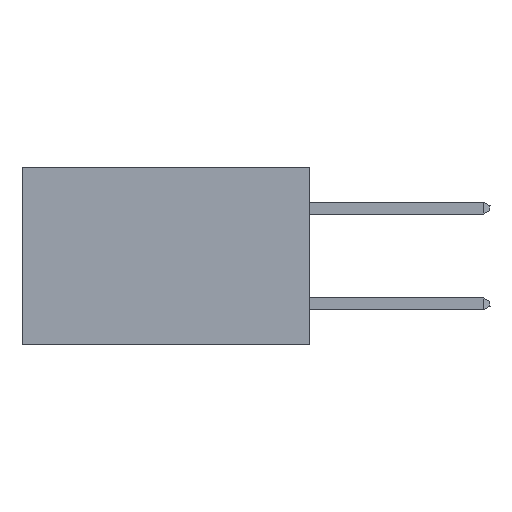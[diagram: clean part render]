
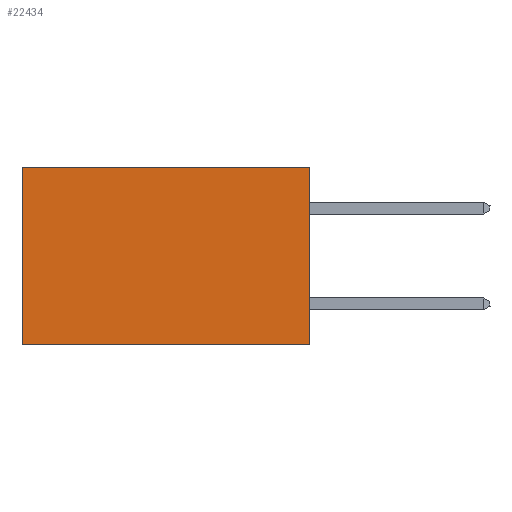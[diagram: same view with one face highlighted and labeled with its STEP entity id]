
A CAD part, left-side view. The second image highlights one B-rep face of the part: STEP entity #22434.
In plain terms, the highlighted planar face has unit normal (-1, 0, 0).
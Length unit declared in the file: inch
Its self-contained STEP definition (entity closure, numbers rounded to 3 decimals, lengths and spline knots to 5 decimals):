
#563 = AXIS2_PLACEMENT_3D ( 'NONE', #19935, #7311, #22118 ) ;
#1279 = CARTESIAN_POINT ( 'NONE',  ( 0.2875, 0.6, 0. ) ) ;
#1547 = DIRECTION ( 'NONE',  ( 0., 0., -1. ) ) ;
#2875 = DIRECTION ( 'NONE',  ( 0., 1., 0. ) ) ;
#2986 = FACE_OUTER_BOUND ( 'NONE', #8673, .T. ) ;
#3261 = LINE ( 'NONE', #4992, #24532 ) ;
#4283 = ORIENTED_EDGE ( 'NONE', *, *, #12725, .F. ) ;
#4875 = CARTESIAN_POINT ( 'NONE',  ( 0.2875, 0., -0.37 ) ) ;
#4992 = CARTESIAN_POINT ( 'NONE',  ( 0.2875, 0., 0. ) ) ;
#5690 = DIRECTION ( 'NONE',  ( 0., 0., -1. ) ) ;
#6287 = CARTESIAN_POINT ( 'NONE',  ( 0.2875, 0., 0. ) ) ;
#6852 = VERTEX_POINT ( 'NONE', #23086 ) ;
#7311 = DIRECTION ( 'NONE',  ( 1., 0., 0. ) ) ;
#7563 = VECTOR ( 'NONE', #5690, 39.37008 ) ;
#8171 = ORIENTED_EDGE ( 'NONE', *, *, #17088, .F. ) ;
#8196 = CARTESIAN_POINT ( 'NONE',  ( 0.2875, 0., 0. ) ) ;
#8673 = EDGE_LOOP ( 'NONE', ( #20246, #4283, #8171, #9065 ) ) ;
#9065 = ORIENTED_EDGE ( 'NONE', *, *, #26227, .T. ) ;
#9244 = CARTESIAN_POINT ( 'NONE',  ( 0.2875, 0., -0.37 ) ) ;
#9646 = VERTEX_POINT ( 'NONE', #6287 ) ;
#10475 = VECTOR ( 'NONE', #19885, 39.37008 ) ;
#12725 = EDGE_CURVE ( 'NONE', #15546, #6852, #16101, .T. ) ;
#13243 = LINE ( 'NONE', #1279, #7563 ) ;
#15546 = VERTEX_POINT ( 'NONE', #4875 ) ;
#16101 = LINE ( 'NONE', #9244, #10475 ) ;
#17088 = EDGE_CURVE ( 'NONE', #9646, #15546, #25831, .T. ) ;
#19885 = DIRECTION ( 'NONE',  ( 0., 1., 0. ) ) ;
#19935 = CARTESIAN_POINT ( 'NONE',  ( 0.2875, 0., 0. ) ) ;
#20246 = ORIENTED_EDGE ( 'NONE', *, *, #23866, .T. ) ;
#20358 = VECTOR ( 'NONE', #1547, 39.37008 ) ;
#21241 = VERTEX_POINT ( 'NONE', #24138 ) ;
#22118 = DIRECTION ( 'NONE',  ( 0., 0., -1. ) ) ;
#22434 = ADVANCED_FACE ( 'NONE', ( #2986 ), #24089, .F. ) ;
#23086 = CARTESIAN_POINT ( 'NONE',  ( 0.2875, 0.6, -0.37 ) ) ;
#23866 = EDGE_CURVE ( 'NONE', #21241, #6852, #13243, .T. ) ;
#24089 = PLANE ( 'NONE',  #563 ) ;
#24138 = CARTESIAN_POINT ( 'NONE',  ( 0.2875, 0.6, 0. ) ) ;
#24532 = VECTOR ( 'NONE', #2875, 39.37008 ) ;
#25831 = LINE ( 'NONE', #8196, #20358 ) ;
#26227 = EDGE_CURVE ( 'NONE', #9646, #21241, #3261, .T. ) ;
